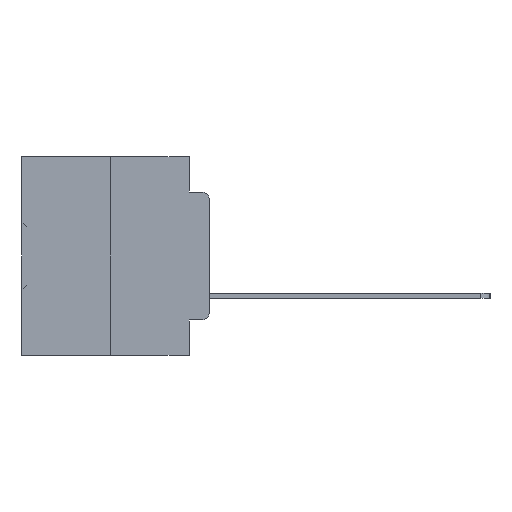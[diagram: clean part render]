
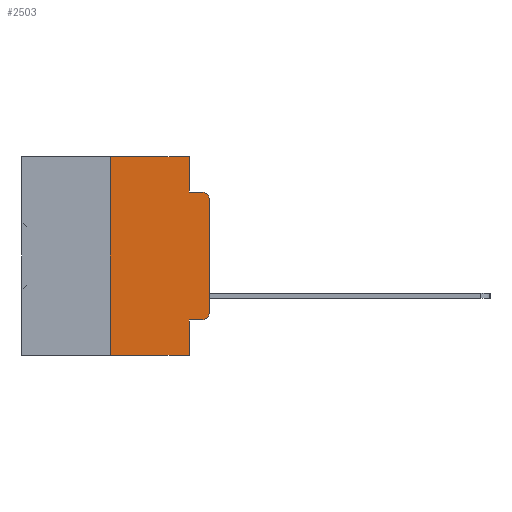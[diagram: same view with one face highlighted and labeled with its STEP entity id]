
A CAD part, left-side view. The second image highlights one B-rep face of the part: STEP entity #2503.
In plain terms, the highlighted planar face has unit normal (-1, 0, 0).
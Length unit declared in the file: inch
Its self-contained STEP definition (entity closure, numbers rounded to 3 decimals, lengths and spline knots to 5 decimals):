
#88 = DIRECTION ( 'NONE',  ( 0., 0., -1. ) ) ;
#175 = EDGE_CURVE ( 'NONE', #33664, #19952, #12198, .T. ) ;
#286 = CIRCLE ( 'NONE', #2307, 0.02 ) ;
#971 = CARTESIAN_POINT ( 'NONE',  ( 0., 0.25, -0.5 ) ) ;
#1085 = VERTEX_POINT ( 'NONE', #30572 ) ;
#1397 = EDGE_CURVE ( 'NONE', #36482, #4790, #2061, .T. ) ;
#2061 = LINE ( 'NONE', #37479, #24474 ) ;
#2307 = AXIS2_PLACEMENT_3D ( 'NONE', #34984, #17728, #88 ) ;
#2420 = DIRECTION ( 'NONE',  ( 1., 0., 0. ) ) ;
#2503 = ADVANCED_FACE ( 'NONE', ( #15265 ), #11082, .F. ) ;
#3315 = DIRECTION ( 'NONE',  ( -1., 0., 0. ) ) ;
#3581 = LINE ( 'NONE', #18831, #25985 ) ;
#4016 = VERTEX_POINT ( 'NONE', #34719 ) ;
#4054 = LINE ( 'NONE', #29494, #12747 ) ;
#4130 = EDGE_CURVE ( 'NONE', #19831, #33664, #4054, .T. ) ;
#4366 = EDGE_CURVE ( 'NONE', #28876, #23122, #3581, .T. ) ;
#4790 = VERTEX_POINT ( 'NONE', #8968 ) ;
#5231 = EDGE_CURVE ( 'NONE', #23122, #1085, #33564, .T. ) ;
#5335 = ORIENTED_EDGE ( 'NONE', *, *, #175, .T. ) ;
#5671 = CARTESIAN_POINT ( 'NONE',  ( 0., 0.051, -0.0885 ) ) ;
#7562 = LINE ( 'NONE', #33328, #29971 ) ;
#8568 = DIRECTION ( 'NONE',  ( 0., -1., 0. ) ) ;
#8904 = ORIENTED_EDGE ( 'NONE', *, *, #16957, .T. ) ;
#8968 = CARTESIAN_POINT ( 'NONE',  ( 0., 0.051, -0.5 ) ) ;
#10031 = EDGE_CURVE ( 'NONE', #31729, #28876, #35884, .T. ) ;
#10322 = ORIENTED_EDGE ( 'NONE', *, *, #4130, .T. ) ;
#10441 = CARTESIAN_POINT ( 'NONE',  ( 0., 0.02, -0.4115 ) ) ;
#10774 = ORIENTED_EDGE ( 'NONE', *, *, #5231, .F. ) ;
#10808 = DIRECTION ( 'NONE',  ( 0., 0., -1. ) ) ;
#11082 = PLANE ( 'NONE',  #36788 ) ;
#11998 = AXIS2_PLACEMENT_3D ( 'NONE', #20946, #3315, #23825 ) ;
#12198 = CIRCLE ( 'NONE', #11998, 0.02 ) ;
#12747 = VECTOR ( 'NONE', #32352, 39.37008 ) ;
#12945 = EDGE_CURVE ( 'NONE', #19952, #4016, #7562, .T. ) ;
#14183 = EDGE_CURVE ( 'NONE', #36482, #31729, #18992, .T. ) ;
#14588 = CARTESIAN_POINT ( 'NONE',  ( 0., 0.051, -0.0885 ) ) ;
#15265 = FACE_OUTER_BOUND ( 'NONE', #31863, .T. ) ;
#15848 = CARTESIAN_POINT ( 'NONE',  ( 0., 0.473, 0. ) ) ;
#15882 = ORIENTED_EDGE ( 'NONE', *, *, #12945, .T. ) ;
#16372 = ORIENTED_EDGE ( 'NONE', *, *, #36718, .F. ) ;
#16957 = EDGE_CURVE ( 'NONE', #4016, #1085, #286, .T. ) ;
#17728 = DIRECTION ( 'NONE',  ( -1., 0., 0. ) ) ;
#18634 = ORIENTED_EDGE ( 'NONE', *, *, #4366, .F. ) ;
#18791 = DIRECTION ( 'NONE',  ( 0., -1., 0. ) ) ;
#18831 = CARTESIAN_POINT ( 'NONE',  ( 0., 0.051, 0. ) ) ;
#18992 = LINE ( 'NONE', #24558, #25772 ) ;
#19831 = VERTEX_POINT ( 'NONE', #24958 ) ;
#19952 = VERTEX_POINT ( 'NONE', #22728 ) ;
#20649 = VECTOR ( 'NONE', #18791, 39.37008 ) ;
#20946 = CARTESIAN_POINT ( 'NONE',  ( 0., 0.02, -0.3915 ) ) ;
#22728 = CARTESIAN_POINT ( 'NONE',  ( 0., 0., -0.3915 ) ) ;
#22891 = CARTESIAN_POINT ( 'NONE',  ( 0., 0.051, 0. ) ) ;
#22936 = DIRECTION ( 'NONE',  ( 0., 0., -1. ) ) ;
#23122 = VERTEX_POINT ( 'NONE', #14588 ) ;
#23825 = DIRECTION ( 'NONE',  ( 0., 0., -1. ) ) ;
#24183 = CARTESIAN_POINT ( 'NONE',  ( 0., 0.25, 0. ) ) ;
#24474 = VECTOR ( 'NONE', #8568, 39.37008 ) ;
#24558 = CARTESIAN_POINT ( 'NONE',  ( 0., 0.25, 0. ) ) ;
#24654 = DIRECTION ( 'NONE',  ( 0., 0., -1. ) ) ;
#24958 = CARTESIAN_POINT ( 'NONE',  ( 0., 0.051, -0.4115 ) ) ;
#25003 = VECTOR ( 'NONE', #10808, 39.37008 ) ;
#25400 = CARTESIAN_POINT ( 'NONE',  ( 0., 0.051, 0. ) ) ;
#25772 = VECTOR ( 'NONE', #33116, 39.37008 ) ;
#25917 = VECTOR ( 'NONE', #34648, 39.37008 ) ;
#25985 = VECTOR ( 'NONE', #24654, 39.37008 ) ;
#26344 = ORIENTED_EDGE ( 'NONE', *, *, #10031, .F. ) ;
#28876 = VERTEX_POINT ( 'NONE', #22891 ) ;
#29494 = CARTESIAN_POINT ( 'NONE',  ( 0., 0.051, -0.4115 ) ) ;
#29971 = VECTOR ( 'NONE', #36158, 39.37008 ) ;
#30572 = CARTESIAN_POINT ( 'NONE',  ( 0., 0.02, -0.0885 ) ) ;
#30878 = ORIENTED_EDGE ( 'NONE', *, *, #1397, .T. ) ;
#31479 = CARTESIAN_POINT ( 'NONE',  ( 0., 0.473, 0. ) ) ;
#31729 = VERTEX_POINT ( 'NONE', #24183 ) ;
#31863 = EDGE_LOOP ( 'NONE', ( #15882, #8904, #10774, #18634, #26344, #35732, #30878, #16372, #10322, #5335 ) ) ;
#32352 = DIRECTION ( 'NONE',  ( 0., -1., 0. ) ) ;
#32671 = LINE ( 'NONE', #25400, #25003 ) ;
#33116 = DIRECTION ( 'NONE',  ( 0., 0., 1. ) ) ;
#33328 = CARTESIAN_POINT ( 'NONE',  ( 0., 0., 0. ) ) ;
#33564 = LINE ( 'NONE', #5671, #25917 ) ;
#33664 = VERTEX_POINT ( 'NONE', #10441 ) ;
#34648 = DIRECTION ( 'NONE',  ( 0., -1., 0. ) ) ;
#34719 = CARTESIAN_POINT ( 'NONE',  ( 0., 0., -0.1085 ) ) ;
#34984 = CARTESIAN_POINT ( 'NONE',  ( 0., 0.02, -0.1085 ) ) ;
#35732 = ORIENTED_EDGE ( 'NONE', *, *, #14183, .F. ) ;
#35884 = LINE ( 'NONE', #15848, #20649 ) ;
#36158 = DIRECTION ( 'NONE',  ( 0., 0., 1. ) ) ;
#36482 = VERTEX_POINT ( 'NONE', #971 ) ;
#36718 = EDGE_CURVE ( 'NONE', #19831, #4790, #32671, .T. ) ;
#36788 = AXIS2_PLACEMENT_3D ( 'NONE', #31479, #2420, #22936 ) ;
#37479 = CARTESIAN_POINT ( 'NONE',  ( 0., 0.473, -0.5 ) ) ;
